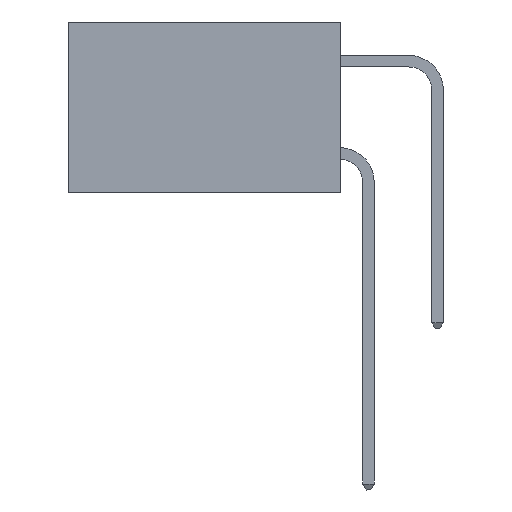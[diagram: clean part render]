
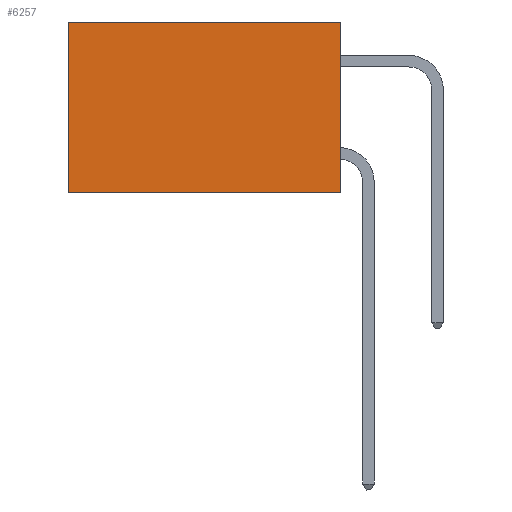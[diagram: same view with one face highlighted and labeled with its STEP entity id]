
A CAD part, left-side view. The second image highlights one B-rep face of the part: STEP entity #6257.
In plain terms, the highlighted planar face has unit normal (-1, 0, 0).
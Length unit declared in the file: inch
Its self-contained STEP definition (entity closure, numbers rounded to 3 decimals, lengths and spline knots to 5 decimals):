
#667 = PLANE ( 'NONE',  #4394 ) ;
#1753 = DIRECTION ( 'NONE',  ( 0., 1., 0. ) ) ;
#2302 = CARTESIAN_POINT ( 'NONE',  ( 0.277, 0., -0.37 ) ) ;
#2519 = VECTOR ( 'NONE', #14250, 39.37008 ) ;
#3825 = VERTEX_POINT ( 'NONE', #9179 ) ;
#3943 = DIRECTION ( 'NONE',  ( 1., 0., 0. ) ) ;
#4394 = AXIS2_PLACEMENT_3D ( 'NONE', #2302, #3943, #14971 ) ;
#4669 = EDGE_CURVE ( 'NONE', #9110, #6961, #7687, .T. ) ;
#4940 = EDGE_CURVE ( 'NONE', #6961, #19372, #6325, .T. ) ;
#5803 = ORIENTED_EDGE ( 'NONE', *, *, #4940, .T. ) ;
#6257 = ADVANCED_FACE ( 'NONE', ( #17665 ), #667, .F. ) ;
#6296 = CARTESIAN_POINT ( 'NONE',  ( 0.277, 0., 0. ) ) ;
#6325 = LINE ( 'NONE', #15231, #16329 ) ;
#6552 = ORIENTED_EDGE ( 'NONE', *, *, #14683, .F. ) ;
#6629 = ORIENTED_EDGE ( 'NONE', *, *, #11612, .F. ) ;
#6691 = ORIENTED_EDGE ( 'NONE', *, *, #4669, .T. ) ;
#6961 = VERTEX_POINT ( 'NONE', #17234 ) ;
#7687 = LINE ( 'NONE', #6296, #19338 ) ;
#9110 = VERTEX_POINT ( 'NONE', #12555 ) ;
#9179 = CARTESIAN_POINT ( 'NONE',  ( 0.277, 0., -0.37 ) ) ;
#10609 = LINE ( 'NONE', #12706, #2519 ) ;
#11612 = EDGE_CURVE ( 'NONE', #9110, #3825, #14165, .T. ) ;
#12555 = CARTESIAN_POINT ( 'NONE',  ( 0.277, 0., 0. ) ) ;
#12706 = CARTESIAN_POINT ( 'NONE',  ( 0.277, 0., -0.37 ) ) ;
#13568 = DIRECTION ( 'NONE',  ( 0., 0., -1. ) ) ;
#14165 = LINE ( 'NONE', #18049, #17237 ) ;
#14250 = DIRECTION ( 'NONE',  ( 0., 1., 0. ) ) ;
#14683 = EDGE_CURVE ( 'NONE', #3825, #19372, #10609, .T. ) ;
#14971 = DIRECTION ( 'NONE',  ( 0., 0., -1. ) ) ;
#15231 = CARTESIAN_POINT ( 'NONE',  ( 0.277, 0.59, -0.37 ) ) ;
#15693 = CARTESIAN_POINT ( 'NONE',  ( 0.277, 0.59, -0.37 ) ) ;
#15722 = EDGE_LOOP ( 'NONE', ( #5803, #6552, #6629, #6691 ) ) ;
#16329 = VECTOR ( 'NONE', #17019, 39.37008 ) ;
#17019 = DIRECTION ( 'NONE',  ( 0., 0., -1. ) ) ;
#17234 = CARTESIAN_POINT ( 'NONE',  ( 0.277, 0.59, 0. ) ) ;
#17237 = VECTOR ( 'NONE', #13568, 39.37008 ) ;
#17665 = FACE_OUTER_BOUND ( 'NONE', #15722, .T. ) ;
#18049 = CARTESIAN_POINT ( 'NONE',  ( 0.277, 0., -0.37 ) ) ;
#19338 = VECTOR ( 'NONE', #1753, 39.37008 ) ;
#19372 = VERTEX_POINT ( 'NONE', #15693 ) ;
